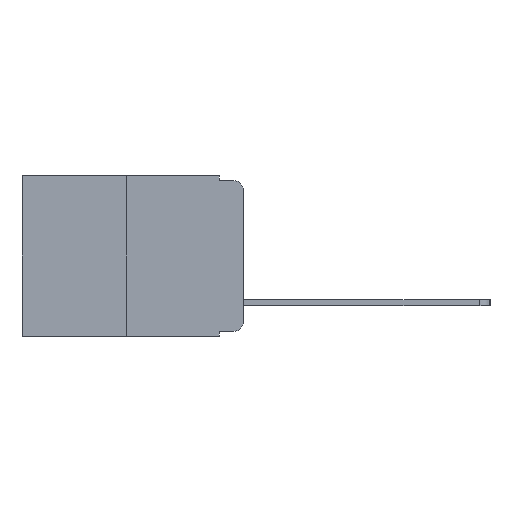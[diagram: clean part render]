
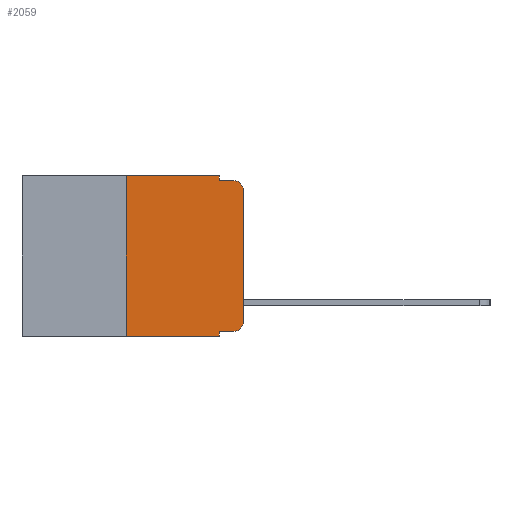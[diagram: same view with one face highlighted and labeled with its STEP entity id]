
A CAD part, left-side view. The second image highlights one B-rep face of the part: STEP entity #2059.
In plain terms, the highlighted planar face has unit normal (-1, 0, 0).
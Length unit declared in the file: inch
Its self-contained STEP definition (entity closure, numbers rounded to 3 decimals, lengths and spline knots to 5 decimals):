
#401 = EDGE_CURVE ( 'NONE', #13534, #10133, #24561, .T. ) ;
#1179 = LINE ( 'NONE', #15397, #21060 ) ;
#1253 = AXIS2_PLACEMENT_3D ( 'NONE', #8563, #21851, #10491 ) ;
#1481 = EDGE_CURVE ( 'NONE', #14387, #10133, #7948, .T. ) ;
#1827 = CARTESIAN_POINT ( 'NONE',  ( 0., 0.051, 0. ) ) ;
#2059 = ADVANCED_FACE ( 'NONE', ( #5487 ), #20098, .F. ) ;
#2369 = CARTESIAN_POINT ( 'NONE',  ( 0., 0., -0.313 ) ) ;
#2401 = CARTESIAN_POINT ( 'NONE',  ( 0., 0.02, -0.03 ) ) ;
#2681 = AXIS2_PLACEMENT_3D ( 'NONE', #19678, #19341, #19290 ) ;
#2715 = VECTOR ( 'NONE', #22946, 39.37008 ) ;
#3191 = VERTEX_POINT ( 'NONE', #14607 ) ;
#3599 = EDGE_CURVE ( 'NONE', #13534, #3191, #12080, .T. ) ;
#3809 = DIRECTION ( 'NONE',  ( 0., 0., -1. ) ) ;
#3926 = DIRECTION ( 'NONE',  ( 0., 0., 1. ) ) ;
#4384 = DIRECTION ( 'NONE',  ( 0., 0., -1. ) ) ;
#4396 = ORIENTED_EDGE ( 'NONE', *, *, #22857, .T. ) ;
#4691 = DIRECTION ( 'NONE',  ( 0., -1., 0. ) ) ;
#4829 = CIRCLE ( 'NONE', #18121, 0.02 ) ;
#4856 = VECTOR ( 'NONE', #4691, 39.37008 ) ;
#5019 = CARTESIAN_POINT ( 'NONE',  ( 0., 0.051, -0.01 ) ) ;
#5487 = FACE_OUTER_BOUND ( 'NONE', #19707, .T. ) ;
#6178 = VECTOR ( 'NONE', #11802, 39.37008 ) ;
#6487 = CARTESIAN_POINT ( 'NONE',  ( 0., 0.02, -0.333 ) ) ;
#6569 = ORIENTED_EDGE ( 'NONE', *, *, #23317, .T. ) ;
#6972 = CARTESIAN_POINT ( 'NONE',  ( 0., 0.25, -0.343 ) ) ;
#7198 = ORIENTED_EDGE ( 'NONE', *, *, #401, .T. ) ;
#7223 = VERTEX_POINT ( 'NONE', #10975 ) ;
#7948 = LINE ( 'NONE', #8648, #2715 ) ;
#8563 = CARTESIAN_POINT ( 'NONE',  ( 0., 0.02, -0.313 ) ) ;
#8625 = CARTESIAN_POINT ( 'NONE',  ( 0., 0., 0. ) ) ;
#8648 = CARTESIAN_POINT ( 'NONE',  ( 0., 0.051, 0. ) ) ;
#9285 = VERTEX_POINT ( 'NONE', #1827 ) ;
#10028 = LINE ( 'NONE', #14380, #4856 ) ;
#10133 = VERTEX_POINT ( 'NONE', #23535 ) ;
#10178 = EDGE_CURVE ( 'NONE', #18673, #20993, #10581, .T. ) ;
#10458 = ORIENTED_EDGE ( 'NONE', *, *, #22866, .T. ) ;
#10491 = DIRECTION ( 'NONE',  ( 0., 0., -1. ) ) ;
#10581 = CIRCLE ( 'NONE', #1253, 0.02 ) ;
#10975 = CARTESIAN_POINT ( 'NONE',  ( 0., 0., -0.03 ) ) ;
#11016 = LINE ( 'NONE', #19283, #6178 ) ;
#11240 = LINE ( 'NONE', #8625, #19565 ) ;
#11802 = DIRECTION ( 'NONE',  ( 0., -1., 0. ) ) ;
#12003 = ORIENTED_EDGE ( 'NONE', *, *, #18510, .F. ) ;
#12080 = LINE ( 'NONE', #13704, #15402 ) ;
#12430 = DIRECTION ( 'NONE',  ( 0., 0., 1. ) ) ;
#12927 = ORIENTED_EDGE ( 'NONE', *, *, #20066, .F. ) ;
#13525 = CARTESIAN_POINT ( 'NONE',  ( 0., 0.051, -0.333 ) ) ;
#13534 = VERTEX_POINT ( 'NONE', #6972 ) ;
#13704 = CARTESIAN_POINT ( 'NONE',  ( 0., 0.25, 0. ) ) ;
#13962 = CARTESIAN_POINT ( 'NONE',  ( 0., 0.02, -0.01 ) ) ;
#14380 = CARTESIAN_POINT ( 'NONE',  ( 0., 0.051, -0.333 ) ) ;
#14387 = VERTEX_POINT ( 'NONE', #13525 ) ;
#14607 = CARTESIAN_POINT ( 'NONE',  ( 0., 0.25, 0. ) ) ;
#15352 = ORIENTED_EDGE ( 'NONE', *, *, #10178, .T. ) ;
#15397 = CARTESIAN_POINT ( 'NONE',  ( 0., 0.051, 0. ) ) ;
#15402 = VECTOR ( 'NONE', #3926, 39.37008 ) ;
#16006 = DIRECTION ( 'NONE',  ( -1., 0., 0. ) ) ;
#16222 = ORIENTED_EDGE ( 'NONE', *, *, #3599, .F. ) ;
#16596 = DIRECTION ( 'NONE',  ( 0., -1., 0. ) ) ;
#17408 = ORIENTED_EDGE ( 'NONE', *, *, #1481, .F. ) ;
#17574 = LINE ( 'NONE', #5019, #18157 ) ;
#17965 = ORIENTED_EDGE ( 'NONE', *, *, #22570, .F. ) ;
#18121 = AXIS2_PLACEMENT_3D ( 'NONE', #2401, #16006, #4384 ) ;
#18157 = VECTOR ( 'NONE', #16596, 39.37008 ) ;
#18510 = EDGE_CURVE ( 'NONE', #3191, #9285, #11016, .T. ) ;
#18646 = CARTESIAN_POINT ( 'NONE',  ( 0., 0.051, -0.01 ) ) ;
#18673 = VERTEX_POINT ( 'NONE', #6487 ) ;
#19079 = VECTOR ( 'NONE', #24482, 39.37008 ) ;
#19283 = CARTESIAN_POINT ( 'NONE',  ( 0., 0.473, 0. ) ) ;
#19290 = DIRECTION ( 'NONE',  ( 0., 0., -1. ) ) ;
#19341 = DIRECTION ( 'NONE',  ( 1., 0., 0. ) ) ;
#19565 = VECTOR ( 'NONE', #12430, 39.37008 ) ;
#19678 = CARTESIAN_POINT ( 'NONE',  ( 0., 0.473, 0. ) ) ;
#19707 = EDGE_LOOP ( 'NONE', ( #10458, #6569, #12927, #17965, #12003, #16222, #7198, #17408, #4396, #15352 ) ) ;
#19802 = VERTEX_POINT ( 'NONE', #13962 ) ;
#20066 = EDGE_CURVE ( 'NONE', #24717, #19802, #17574, .T. ) ;
#20098 = PLANE ( 'NONE',  #2681 ) ;
#20993 = VERTEX_POINT ( 'NONE', #2369 ) ;
#21060 = VECTOR ( 'NONE', #3809, 39.37008 ) ;
#21851 = DIRECTION ( 'NONE',  ( -1., 0., 0. ) ) ;
#22570 = EDGE_CURVE ( 'NONE', #9285, #24717, #1179, .T. ) ;
#22857 = EDGE_CURVE ( 'NONE', #14387, #18673, #10028, .T. ) ;
#22866 = EDGE_CURVE ( 'NONE', #20993, #7223, #11240, .T. ) ;
#22946 = DIRECTION ( 'NONE',  ( 0., 0., -1. ) ) ;
#23317 = EDGE_CURVE ( 'NONE', #7223, #19802, #4829, .T. ) ;
#23535 = CARTESIAN_POINT ( 'NONE',  ( 0., 0.051, -0.343 ) ) ;
#24456 = CARTESIAN_POINT ( 'NONE',  ( 0., 0.473, -0.343 ) ) ;
#24482 = DIRECTION ( 'NONE',  ( 0., -1., 0. ) ) ;
#24561 = LINE ( 'NONE', #24456, #19079 ) ;
#24717 = VERTEX_POINT ( 'NONE', #18646 ) ;
